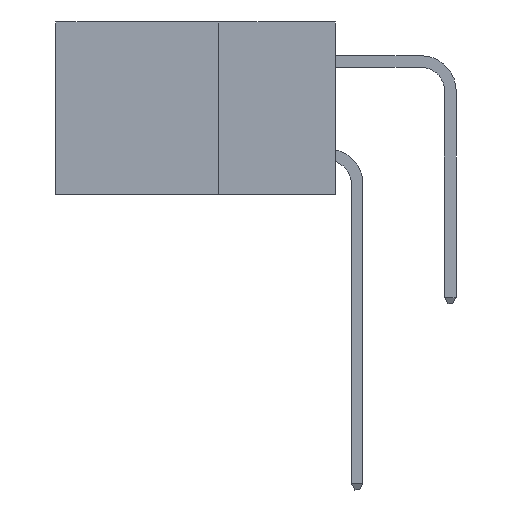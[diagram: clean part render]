
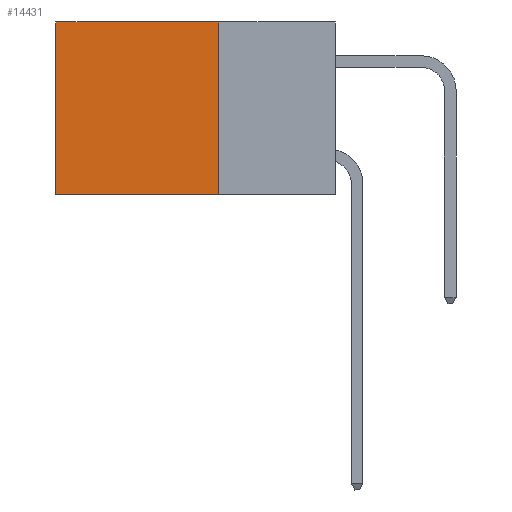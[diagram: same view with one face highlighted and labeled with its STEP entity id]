
A CAD part, left-side view. The second image highlights one B-rep face of the part: STEP entity #14431.
In plain terms, the highlighted planar face has unit normal (-1, 0, 0).
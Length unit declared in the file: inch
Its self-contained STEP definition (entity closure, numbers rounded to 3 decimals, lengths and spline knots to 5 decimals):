
#1817 = CARTESIAN_POINT ( 'NONE',  ( 0.2875, 0.25, -0.37 ) ) ;
#2773 = LINE ( 'NONE', #36443, #24663 ) ;
#5942 = CARTESIAN_POINT ( 'NONE',  ( 0.2875, 0.25, 0. ) ) ;
#6051 = DIRECTION ( 'NONE',  ( 1., 0., 0. ) ) ;
#6469 = VERTEX_POINT ( 'NONE', #21923 ) ;
#6958 = DIRECTION ( 'NONE',  ( 0., 1., 0. ) ) ;
#7509 = VERTEX_POINT ( 'NONE', #15272 ) ;
#9705 = ORIENTED_EDGE ( 'NONE', *, *, #39918, .T. ) ;
#12383 = CARTESIAN_POINT ( 'NONE',  ( 0.2875, 0.25, 0. ) ) ;
#13417 = DIRECTION ( 'NONE',  ( 0., 1., 0. ) ) ;
#14431 = ADVANCED_FACE ( 'NONE', ( #23280 ), #28927, .F. ) ;
#14610 = ORIENTED_EDGE ( 'NONE', *, *, #19432, .F. ) ;
#15272 = CARTESIAN_POINT ( 'NONE',  ( 0.2875, 0.25, 0. ) ) ;
#16348 = VERTEX_POINT ( 'NONE', #1817 ) ;
#16426 = AXIS2_PLACEMENT_3D ( 'NONE', #25616, #6051, #32226 ) ;
#17034 = DIRECTION ( 'NONE',  ( 0., 0., -1. ) ) ;
#17641 = ORIENTED_EDGE ( 'NONE', *, *, #36920, .F. ) ;
#19432 = EDGE_CURVE ( 'NONE', #7509, #16348, #42000, .T. ) ;
#19994 = VERTEX_POINT ( 'NONE', #25849 ) ;
#21923 = CARTESIAN_POINT ( 'NONE',  ( 0.2875, 0.6, 0. ) ) ;
#23032 = LINE ( 'NONE', #12383, #23530 ) ;
#23280 = FACE_OUTER_BOUND ( 'NONE', #39790, .T. ) ;
#23530 = VECTOR ( 'NONE', #6958, 39.37008 ) ;
#24663 = VECTOR ( 'NONE', #13417, 39.37008 ) ;
#25360 = DIRECTION ( 'NONE',  ( 0., 0., -1. ) ) ;
#25616 = CARTESIAN_POINT ( 'NONE',  ( 0.2875, 0.25, 0. ) ) ;
#25849 = CARTESIAN_POINT ( 'NONE',  ( 0.2875, 0.6, -0.37 ) ) ;
#26789 = CARTESIAN_POINT ( 'NONE',  ( 0.2875, 0.6, 0. ) ) ;
#28927 = PLANE ( 'NONE',  #16426 ) ;
#31506 = EDGE_CURVE ( 'NONE', #7509, #6469, #23032, .T. ) ;
#32226 = DIRECTION ( 'NONE',  ( 0., 0., -1. ) ) ;
#32315 = VECTOR ( 'NONE', #25360, 39.37008 ) ;
#33171 = VECTOR ( 'NONE', #17034, 39.37008 ) ;
#34269 = ORIENTED_EDGE ( 'NONE', *, *, #31506, .T. ) ;
#36443 = CARTESIAN_POINT ( 'NONE',  ( 0.2875, 0.25, -0.37 ) ) ;
#36920 = EDGE_CURVE ( 'NONE', #16348, #19994, #2773, .T. ) ;
#39790 = EDGE_LOOP ( 'NONE', ( #9705, #17641, #14610, #34269 ) ) ;
#39918 = EDGE_CURVE ( 'NONE', #6469, #19994, #41348, .T. ) ;
#41348 = LINE ( 'NONE', #26789, #33171 ) ;
#42000 = LINE ( 'NONE', #5942, #32315 ) ;
